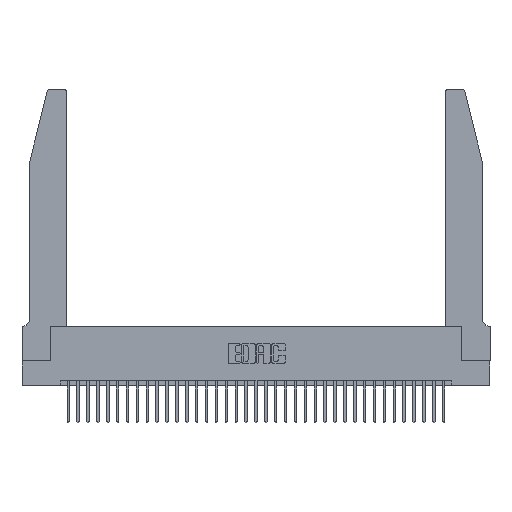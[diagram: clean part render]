
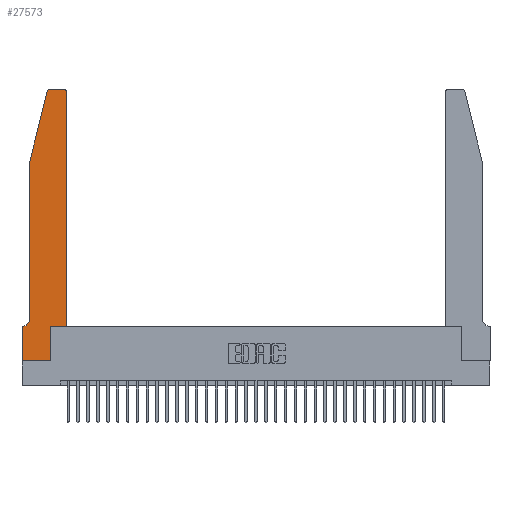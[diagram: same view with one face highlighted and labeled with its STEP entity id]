
A CAD part, top view. The second image highlights one B-rep face of the part: STEP entity #27573.
In plain terms, the highlighted planar face has unit normal (0, 0, 1).
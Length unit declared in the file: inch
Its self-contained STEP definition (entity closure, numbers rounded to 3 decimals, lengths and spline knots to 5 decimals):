
#545 = CARTESIAN_POINT ( 'NONE',  ( 0.0755, 2., 0.37 ) ) ;
#957 = EDGE_CURVE ( 'NONE', #20899, #10183, #3644, .T. ) ;
#1076 = EDGE_CURVE ( 'NONE', #10183, #24092, #4076, .T. ) ;
#1538 = CARTESIAN_POINT ( 'NONE',  ( 0.4505, 0.35, 0.37 ) ) ;
#1560 = CARTESIAN_POINT ( 'NONE',  ( 0., 0.35, 0.37 ) ) ;
#1985 = DIRECTION ( 'NONE',  ( -1., 0., 0. ) ) ;
#2321 = VERTEX_POINT ( 'NONE', #32604 ) ;
#2511 = CARTESIAN_POINT ( 'NONE',  ( 0.4505, 0.35, 0.37 ) ) ;
#2635 = DIRECTION ( 'NONE',  ( 1., 0., 0. ) ) ;
#3119 = ORIENTED_EDGE ( 'NONE', *, *, #8620, .T. ) ;
#3339 = PLANE ( 'NONE',  #29234 ) ;
#3455 = DIRECTION ( 'NONE',  ( -1., 0., 0. ) ) ;
#3552 = EDGE_CURVE ( 'NONE', #27537, #13600, #8770, .T. ) ;
#3644 = LINE ( 'NONE', #30736, #21367 ) ;
#3719 = CIRCLE ( 'NONE', #14738, 0.03 ) ;
#3780 = CARTESIAN_POINT ( 'NONE',  ( 0.2865, 0.35, 0.37 ) ) ;
#3791 = CARTESIAN_POINT ( 'NONE',  ( 0.2865, 0.35, 0.37 ) ) ;
#3901 = DIRECTION ( 'NONE',  ( 0., 1., 0. ) ) ;
#4076 = LINE ( 'NONE', #27740, #5784 ) ;
#5258 = ORIENTED_EDGE ( 'NONE', *, *, #11059, .T. ) ;
#5446 = DIRECTION ( 'NONE',  ( 1., 0., 0. ) ) ;
#5784 = VECTOR ( 'NONE', #33991, 39.37008 ) ;
#6489 = CARTESIAN_POINT ( 'NONE',  ( 0.284, 2.75, 0.37 ) ) ;
#6665 = VECTOR ( 'NONE', #2635, 39.37008 ) ;
#6980 = VECTOR ( 'NONE', #33455, 39.37008 ) ;
#7816 = CARTESIAN_POINT ( 'NONE',  ( 0.4505, 2.72, 0.37 ) ) ;
#8620 = EDGE_CURVE ( 'NONE', #10351, #32748, #23609, .T. ) ;
#8707 = ORIENTED_EDGE ( 'NONE', *, *, #34392, .T. ) ;
#8770 = LINE ( 'NONE', #3791, #30027 ) ;
#9098 = EDGE_CURVE ( 'NONE', #24092, #27537, #27201, .T. ) ;
#10183 = VERTEX_POINT ( 'NONE', #1560 ) ;
#10351 = VERTEX_POINT ( 'NONE', #31213 ) ;
#11059 = EDGE_CURVE ( 'NONE', #13600, #11235, #12225, .T. ) ;
#11067 = ORIENTED_EDGE ( 'NONE', *, *, #11728, .T. ) ;
#11235 = VERTEX_POINT ( 'NONE', #1538 ) ;
#11594 = LINE ( 'NONE', #35716, #26369 ) ;
#11724 = EDGE_CURVE ( 'NONE', #22967, #25240, #22608, .T. ) ;
#11728 = EDGE_CURVE ( 'NONE', #11235, #22967, #21786, .T. ) ;
#11843 = ORIENTED_EDGE ( 'NONE', *, *, #19265, .T. ) ;
#12153 = DIRECTION ( 'NONE',  ( 0., 0., 1. ) ) ;
#12225 = LINE ( 'NONE', #2511, #6665 ) ;
#12533 = CARTESIAN_POINT ( 'NONE',  ( 0.4205, 2.72, 0.37 ) ) ;
#12582 = CARTESIAN_POINT ( 'NONE',  ( 0.4205, 2.75, 0.37 ) ) ;
#13461 = LINE ( 'NONE', #545, #6980 ) ;
#13545 = VECTOR ( 'NONE', #3901, 39.37008 ) ;
#13600 = VERTEX_POINT ( 'NONE', #3780 ) ;
#14738 = AXIS2_PLACEMENT_3D ( 'NONE', #15392, #23993, #18062 ) ;
#15392 = CARTESIAN_POINT ( 'NONE',  ( 0.284, 2.72, 0.37 ) ) ;
#15606 = CARTESIAN_POINT ( 'NONE',  ( 0.0055, 0.42, 0.37 ) ) ;
#17125 = FACE_OUTER_BOUND ( 'NONE', #17197, .T. ) ;
#17197 = EDGE_LOOP ( 'NONE', ( #11843, #8707, #3119, #22976, #26169, #29711, #35170, #35351, #19284, #5258, #11067, #17516 ) ) ;
#17380 = EDGE_CURVE ( 'NONE', #32748, #2321, #13461, .T. ) ;
#17516 = ORIENTED_EDGE ( 'NONE', *, *, #11724, .T. ) ;
#18062 = DIRECTION ( 'NONE',  ( 1., 0., 0. ) ) ;
#18308 = CARTESIAN_POINT ( 'NONE',  ( 0.0755, 2., 0.37 ) ) ;
#18539 = DIRECTION ( 'NONE',  ( 0., 0., -1. ) ) ;
#19265 = EDGE_CURVE ( 'NONE', #25240, #33689, #11594, .T. ) ;
#19284 = ORIENTED_EDGE ( 'NONE', *, *, #3552, .T. ) ;
#19533 = AXIS2_PLACEMENT_3D ( 'NONE', #15606, #18539, #1985 ) ;
#19644 = DIRECTION ( 'NONE',  ( 1., 0., 0. ) ) ;
#19967 = EDGE_CURVE ( 'NONE', #2321, #20899, #28887, .T. ) ;
#20899 = VERTEX_POINT ( 'NONE', #27834 ) ;
#21241 = AXIS2_PLACEMENT_3D ( 'NONE', #12533, #12153, #34584 ) ;
#21367 = VECTOR ( 'NONE', #3455, 39.37008 ) ;
#21627 = CARTESIAN_POINT ( 'NONE',  ( 0.2865, 0., 0.37 ) ) ;
#21786 = LINE ( 'NONE', #26094, #13545 ) ;
#21986 = CARTESIAN_POINT ( 'NONE',  ( 0., 0., 0.37 ) ) ;
#22138 = CARTESIAN_POINT ( 'NONE',  ( 0., 0., 0.37 ) ) ;
#22608 = CIRCLE ( 'NONE', #21241, 0.03 ) ;
#22967 = VERTEX_POINT ( 'NONE', #7816 ) ;
#22976 = ORIENTED_EDGE ( 'NONE', *, *, #17380, .T. ) ;
#23114 = CARTESIAN_POINT ( 'NONE',  ( 0.0755, 2., 0.37 ) ) ;
#23609 = LINE ( 'NONE', #23114, #26195 ) ;
#23993 = DIRECTION ( 'NONE',  ( 0., 0., 1. ) ) ;
#24092 = VERTEX_POINT ( 'NONE', #22138 ) ;
#25240 = VERTEX_POINT ( 'NONE', #12582 ) ;
#26094 = CARTESIAN_POINT ( 'NONE',  ( 0.4505, 0.35, 0.37 ) ) ;
#26169 = ORIENTED_EDGE ( 'NONE', *, *, #19967, .T. ) ;
#26195 = VECTOR ( 'NONE', #31087, 39.37008 ) ;
#26369 = VECTOR ( 'NONE', #26431, 39.37008 ) ;
#26431 = DIRECTION ( 'NONE',  ( -1., 0., 0. ) ) ;
#27201 = LINE ( 'NONE', #21986, #29748 ) ;
#27537 = VERTEX_POINT ( 'NONE', #21627 ) ;
#27573 = ADVANCED_FACE ( 'NONE', ( #17125 ), #3339, .T. ) ;
#27740 = CARTESIAN_POINT ( 'NONE',  ( 0., 0., 0.37 ) ) ;
#27834 = CARTESIAN_POINT ( 'NONE',  ( 0.0055, 0.35, 0.37 ) ) ;
#28887 = CIRCLE ( 'NONE', #19533, 0.07 ) ;
#29234 = AXIS2_PLACEMENT_3D ( 'NONE', #33648, #33308, #19644 ) ;
#29711 = ORIENTED_EDGE ( 'NONE', *, *, #957, .T. ) ;
#29748 = VECTOR ( 'NONE', #5446, 39.37008 ) ;
#30027 = VECTOR ( 'NONE', #33496, 39.37008 ) ;
#30736 = CARTESIAN_POINT ( 'NONE',  ( 0.0755, 0.35, 0.37 ) ) ;
#31087 = DIRECTION ( 'NONE',  ( -0.239, -0.971, 0. ) ) ;
#31213 = CARTESIAN_POINT ( 'NONE',  ( 0.25487, 2.72718, 0.37 ) ) ;
#32604 = CARTESIAN_POINT ( 'NONE',  ( 0.0755, 0.42, 0.37 ) ) ;
#32748 = VERTEX_POINT ( 'NONE', #18308 ) ;
#33308 = DIRECTION ( 'NONE',  ( 0., 0., 1. ) ) ;
#33455 = DIRECTION ( 'NONE',  ( 0., -1., 0. ) ) ;
#33496 = DIRECTION ( 'NONE',  ( 0., 1., 0. ) ) ;
#33648 = CARTESIAN_POINT ( 'NONE',  ( 0., 0.35, 0.37 ) ) ;
#33689 = VERTEX_POINT ( 'NONE', #6489 ) ;
#33991 = DIRECTION ( 'NONE',  ( 0., -1., 0. ) ) ;
#34392 = EDGE_CURVE ( 'NONE', #33689, #10351, #3719, .T. ) ;
#34584 = DIRECTION ( 'NONE',  ( 1., 0., 0. ) ) ;
#35170 = ORIENTED_EDGE ( 'NONE', *, *, #1076, .T. ) ;
#35351 = ORIENTED_EDGE ( 'NONE', *, *, #9098, .T. ) ;
#35716 = CARTESIAN_POINT ( 'NONE',  ( 0.2605, 2.75, 0.37 ) ) ;
